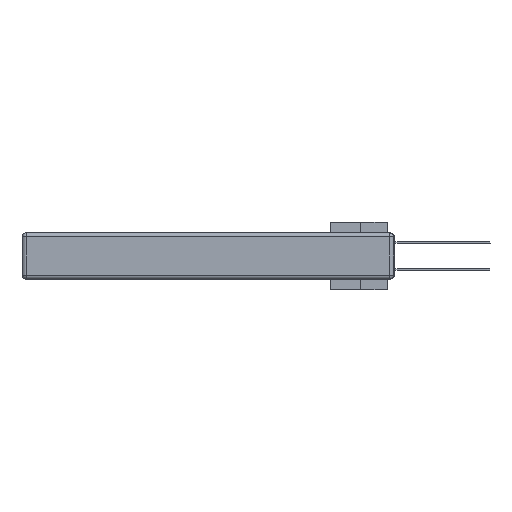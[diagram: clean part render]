
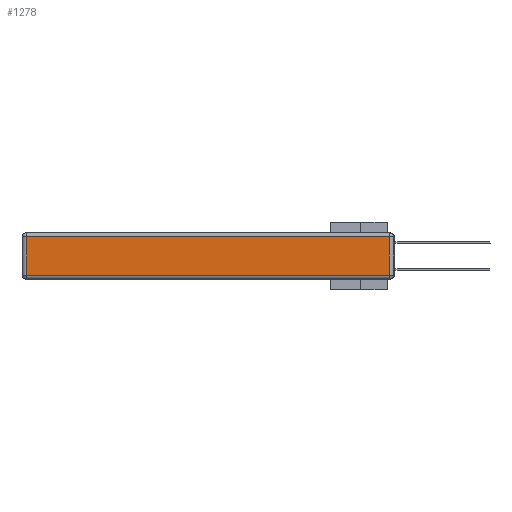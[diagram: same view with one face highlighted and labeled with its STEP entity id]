
A CAD part, left-side view. The second image highlights one B-rep face of the part: STEP entity #1278.
In plain terms, the highlighted planar face has unit normal (-1, 0, 0).
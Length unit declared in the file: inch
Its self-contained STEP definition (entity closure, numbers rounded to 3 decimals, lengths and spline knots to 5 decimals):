
#123 = DIRECTION ( 'NONE',  ( -1., 0., 0. ) ) ;
#614 = DIRECTION ( 'NONE',  ( 0., 1., 0. ) ) ;
#1195 = ORIENTED_EDGE ( 'NONE', *, *, #28444, .T. ) ;
#1278 = ADVANCED_FACE ( 'NONE', ( #2881 ), #20992, .T. ) ;
#2869 = CARTESIAN_POINT ( 'NONE',  ( 0., 2.72, -0.03 ) ) ;
#2881 = FACE_OUTER_BOUND ( 'NONE', #31685, .T. ) ;
#3612 = ORIENTED_EDGE ( 'NONE', *, *, #9558, .T. ) ;
#5261 = EDGE_CURVE ( 'NONE', #10803, #19865, #14233, .T. ) ;
#7356 = VERTEX_POINT ( 'NONE', #32882 ) ;
#8799 = VECTOR ( 'NONE', #24291, 39.37008 ) ;
#8891 = VECTOR ( 'NONE', #32966, 39.37008 ) ;
#9459 = LINE ( 'NONE', #9615, #8891 ) ;
#9558 = EDGE_CURVE ( 'NONE', #7356, #24457, #22205, .T. ) ;
#9615 = CARTESIAN_POINT ( 'NONE',  ( 0., 0.03, -0.343 ) ) ;
#10803 = VERTEX_POINT ( 'NONE', #15517 ) ;
#10852 = ORIENTED_EDGE ( 'NONE', *, *, #18010, .T. ) ;
#12738 = CARTESIAN_POINT ( 'NONE',  ( 0., 0., -0.343 ) ) ;
#12753 = ORIENTED_EDGE ( 'NONE', *, *, #5261, .T. ) ;
#14233 = LINE ( 'NONE', #24236, #33345 ) ;
#15517 = CARTESIAN_POINT ( 'NONE',  ( 0., 0.03, -0.03 ) ) ;
#17439 = AXIS2_PLACEMENT_3D ( 'NONE', #12738, #123, #18400 ) ;
#18010 = EDGE_CURVE ( 'NONE', #19865, #7356, #32297, .T. ) ;
#18400 = DIRECTION ( 'NONE',  ( 0., 0., 1. ) ) ;
#19865 = VERTEX_POINT ( 'NONE', #2869 ) ;
#20992 = PLANE ( 'NONE',  #17439 ) ;
#21150 = CARTESIAN_POINT ( 'NONE',  ( 0., 0.03, -0.313 ) ) ;
#22205 = LINE ( 'NONE', #32631, #8799 ) ;
#24236 = CARTESIAN_POINT ( 'NONE',  ( 0., 2.75, -0.03 ) ) ;
#24291 = DIRECTION ( 'NONE',  ( 0., -1., 0. ) ) ;
#24457 = VERTEX_POINT ( 'NONE', #21150 ) ;
#26652 = DIRECTION ( 'NONE',  ( 0., 0., -1. ) ) ;
#28444 = EDGE_CURVE ( 'NONE', #24457, #10803, #9459, .T. ) ;
#29003 = VECTOR ( 'NONE', #26652, 39.37008 ) ;
#31685 = EDGE_LOOP ( 'NONE', ( #3612, #1195, #12753, #10852 ) ) ;
#32126 = CARTESIAN_POINT ( 'NONE',  ( 0., 2.72, -0.343 ) ) ;
#32297 = LINE ( 'NONE', #32126, #29003 ) ;
#32631 = CARTESIAN_POINT ( 'NONE',  ( 0., 0., -0.313 ) ) ;
#32882 = CARTESIAN_POINT ( 'NONE',  ( 0., 2.72, -0.313 ) ) ;
#32966 = DIRECTION ( 'NONE',  ( 0., 0., 1. ) ) ;
#33345 = VECTOR ( 'NONE', #614, 39.37008 ) ;
